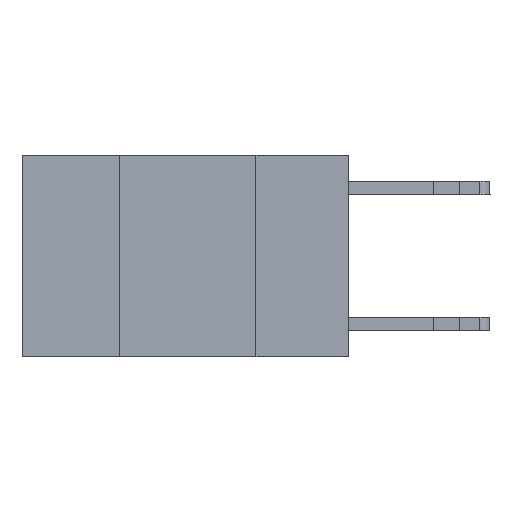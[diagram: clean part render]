
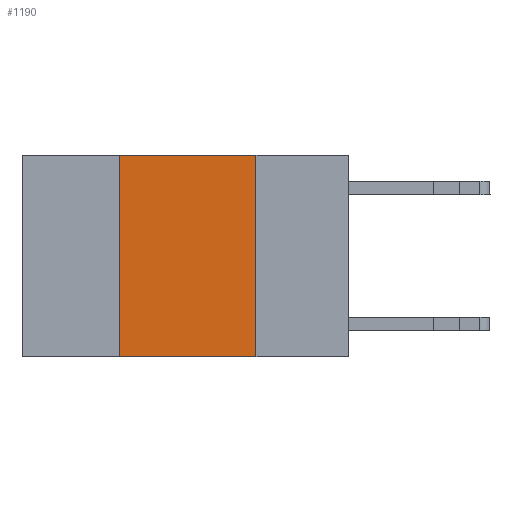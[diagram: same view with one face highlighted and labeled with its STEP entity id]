
A CAD part, left-side view. The second image highlights one B-rep face of the part: STEP entity #1190.
In plain terms, the highlighted planar face has unit normal (-1, 0, 0).
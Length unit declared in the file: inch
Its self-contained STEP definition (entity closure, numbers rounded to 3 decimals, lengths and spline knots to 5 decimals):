
#377 = VERTEX_POINT ( 'NONE', #14419 ) ;
#914 = VECTOR ( 'NONE', #3449, 39.37008 ) ;
#1016 = VECTOR ( 'NONE', #19114, 39.37008 ) ;
#1055 = LINE ( 'NONE', #6691, #914 ) ;
#1153 = DIRECTION ( 'NONE',  ( 0., 0., -1. ) ) ;
#1166 = LINE ( 'NONE', #19233, #1016 ) ;
#1190 = ADVANCED_FACE ( 'NONE', ( #11006 ), #3268, .F. ) ;
#2563 = VERTEX_POINT ( 'NONE', #9096 ) ;
#2587 = EDGE_LOOP ( 'NONE', ( #14217, #13845, #13908, #20208 ) ) ;
#3268 = PLANE ( 'NONE',  #15910 ) ;
#3449 = DIRECTION ( 'NONE',  ( 0., -1., 0. ) ) ;
#3820 = EDGE_CURVE ( 'NONE', #377, #17030, #11097, .T. ) ;
#4362 = CARTESIAN_POINT ( 'NONE',  ( 0., 0.17, 0. ) ) ;
#5474 = DIRECTION ( 'NONE',  ( 0., 0., 1. ) ) ;
#5517 = CARTESIAN_POINT ( 'NONE',  ( 0., 0.42, 0. ) ) ;
#6691 = CARTESIAN_POINT ( 'NONE',  ( 0., 0.6, 0. ) ) ;
#6878 = VERTEX_POINT ( 'NONE', #13274 ) ;
#9096 = CARTESIAN_POINT ( 'NONE',  ( 0., 0.17, -0.37 ) ) ;
#11006 = FACE_OUTER_BOUND ( 'NONE', #2587, .T. ) ;
#11097 = LINE ( 'NONE', #5517, #11226 ) ;
#11226 = VECTOR ( 'NONE', #5474, 39.37008 ) ;
#13100 = CARTESIAN_POINT ( 'NONE',  ( 0., 0.42, 0. ) ) ;
#13274 = CARTESIAN_POINT ( 'NONE',  ( 0., 0.17, 0. ) ) ;
#13845 = ORIENTED_EDGE ( 'NONE', *, *, #19714, .F. ) ;
#13908 = ORIENTED_EDGE ( 'NONE', *, *, #3820, .F. ) ;
#14050 = DIRECTION ( 'NONE',  ( 1., 0., 0. ) ) ;
#14217 = ORIENTED_EDGE ( 'NONE', *, *, #14645, .F. ) ;
#14277 = EDGE_CURVE ( 'NONE', #377, #2563, #1166, .T. ) ;
#14419 = CARTESIAN_POINT ( 'NONE',  ( 0., 0.42, -0.37 ) ) ;
#14645 = EDGE_CURVE ( 'NONE', #6878, #2563, #19555, .T. ) ;
#15210 = CARTESIAN_POINT ( 'NONE',  ( 0., 0.6, 0. ) ) ;
#15910 = AXIS2_PLACEMENT_3D ( 'NONE', #15210, #14050, #19410 ) ;
#17030 = VERTEX_POINT ( 'NONE', #13100 ) ;
#19114 = DIRECTION ( 'NONE',  ( 0., -1., 0. ) ) ;
#19233 = CARTESIAN_POINT ( 'NONE',  ( 0., 0.6, -0.37 ) ) ;
#19309 = VECTOR ( 'NONE', #1153, 39.37008 ) ;
#19410 = DIRECTION ( 'NONE',  ( 0., 0., -1. ) ) ;
#19555 = LINE ( 'NONE', #4362, #19309 ) ;
#19714 = EDGE_CURVE ( 'NONE', #17030, #6878, #1055, .T. ) ;
#20208 = ORIENTED_EDGE ( 'NONE', *, *, #14277, .T. ) ;
